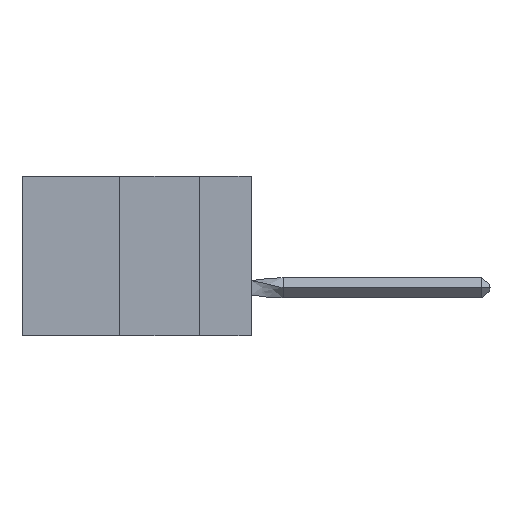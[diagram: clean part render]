
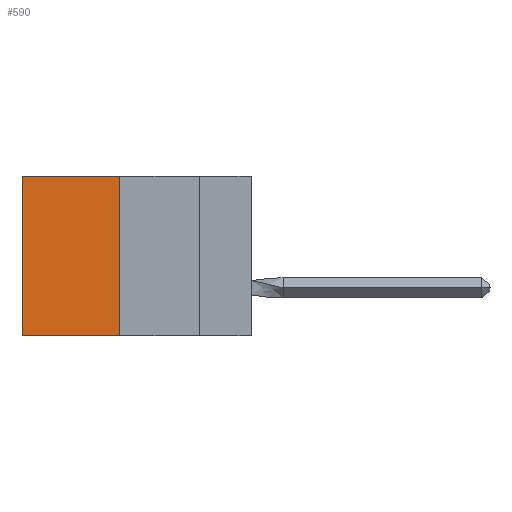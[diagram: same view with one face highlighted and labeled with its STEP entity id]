
A CAD part, left-side view. The second image highlights one B-rep face of the part: STEP entity #590.
In plain terms, the highlighted planar face has unit normal (-1, 0, 0).
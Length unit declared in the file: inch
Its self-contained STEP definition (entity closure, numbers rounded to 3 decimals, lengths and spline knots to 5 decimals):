
#21 = EDGE_CURVE ( 'NONE', #3654, #15591, #6428, .T. ) ;
#432 = LINE ( 'NONE', #1775, #13725 ) ;
#445 = DIRECTION ( 'NONE',  ( 0., 1., 0. ) ) ;
#590 = ADVANCED_FACE ( 'NONE', ( #11905 ), #8267, .F. ) ;
#665 = DIRECTION ( 'NONE',  ( 0., 0., -1. ) ) ;
#840 = VECTOR ( 'NONE', #445, 39.37008 ) ;
#1678 = DIRECTION ( 'NONE',  ( 0., 0., -1. ) ) ;
#1775 = CARTESIAN_POINT ( 'NONE',  ( 0.305, 0.413, 0. ) ) ;
#1891 = LINE ( 'NONE', #9830, #840 ) ;
#1998 = CARTESIAN_POINT ( 'NONE',  ( 0.305, 0.413, -0.5 ) ) ;
#2267 = EDGE_CURVE ( 'NONE', #15591, #17057, #1891, .T. ) ;
#3049 = EDGE_CURVE ( 'NONE', #13402, #17057, #10963, .T. ) ;
#3143 = DIRECTION ( 'NONE',  ( 0., 1., 0. ) ) ;
#3654 = VERTEX_POINT ( 'NONE', #14358 ) ;
#3693 = ORIENTED_EDGE ( 'NONE', *, *, #2267, .F. ) ;
#3893 = AXIS2_PLACEMENT_3D ( 'NONE', #13805, #9788, #1678 ) ;
#4012 = VECTOR ( 'NONE', #665, 39.37008 ) ;
#4330 = DIRECTION ( 'NONE',  ( 0., 0., -1. ) ) ;
#6428 = LINE ( 'NONE', #10937, #9179 ) ;
#6647 = CARTESIAN_POINT ( 'NONE',  ( 0.305, 0.72, -0.5 ) ) ;
#8267 = PLANE ( 'NONE',  #3893 ) ;
#8413 = ORIENTED_EDGE ( 'NONE', *, *, #21, .F. ) ;
#8452 = CARTESIAN_POINT ( 'NONE',  ( 0.305, 0.72, 0. ) ) ;
#8938 = CARTESIAN_POINT ( 'NONE',  ( 0.305, 0.72, -0.5 ) ) ;
#9179 = VECTOR ( 'NONE', #4330, 39.37008 ) ;
#9232 = ORIENTED_EDGE ( 'NONE', *, *, #3049, .T. ) ;
#9788 = DIRECTION ( 'NONE',  ( 1., 0., 0. ) ) ;
#9830 = CARTESIAN_POINT ( 'NONE',  ( 0.305, 0.413, -0.5 ) ) ;
#9926 = EDGE_CURVE ( 'NONE', #3654, #13402, #432, .T. ) ;
#10693 = ORIENTED_EDGE ( 'NONE', *, *, #9926, .T. ) ;
#10937 = CARTESIAN_POINT ( 'NONE',  ( 0.305, 0.413, -0.5 ) ) ;
#10963 = LINE ( 'NONE', #8938, #4012 ) ;
#11905 = FACE_OUTER_BOUND ( 'NONE', #14242, .T. ) ;
#13402 = VERTEX_POINT ( 'NONE', #8452 ) ;
#13725 = VECTOR ( 'NONE', #3143, 39.37008 ) ;
#13805 = CARTESIAN_POINT ( 'NONE',  ( 0.305, 0.413, -0.5 ) ) ;
#14242 = EDGE_LOOP ( 'NONE', ( #9232, #3693, #8413, #10693 ) ) ;
#14358 = CARTESIAN_POINT ( 'NONE',  ( 0.305, 0.413, 0. ) ) ;
#15591 = VERTEX_POINT ( 'NONE', #1998 ) ;
#17057 = VERTEX_POINT ( 'NONE', #6647 ) ;
